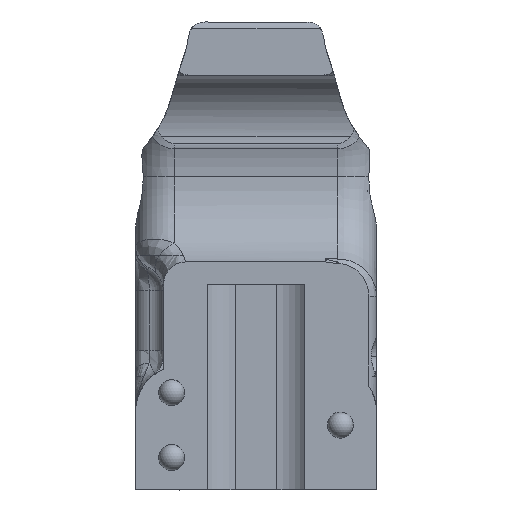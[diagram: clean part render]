
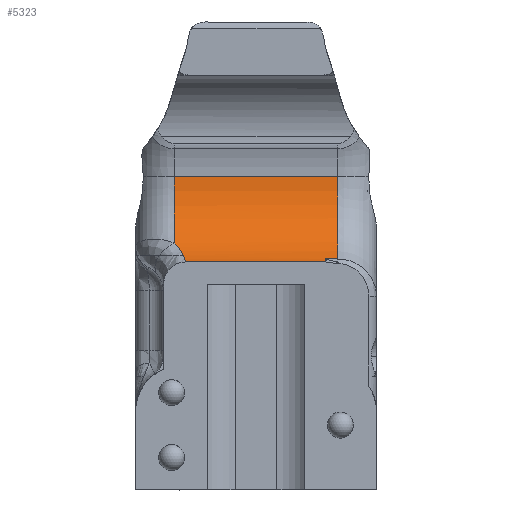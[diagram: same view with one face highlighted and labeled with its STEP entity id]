
A CAD part, left-side view. The second image highlights one B-rep face of the part: STEP entity #5323.
In plain terms, the highlighted cylindrical face has radius 14.287 mm (diameter 28.575 mm), a partial arc.
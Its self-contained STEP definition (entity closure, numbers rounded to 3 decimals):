
#4 = CARTESIAN_POINT ( 'NONE',  ( 76.653, -72.447, -1.367 ) ) ;
#103 = CARTESIAN_POINT ( 'NONE',  ( 84.171, -46.951, -13.516 ) ) ;
#279 = VERTEX_POINT ( 'NONE', #3053 ) ;
#500 = ORIENTED_EDGE ( 'NONE', *, *, #2014, .T. ) ;
#787 = CARTESIAN_POINT ( 'NONE',  ( 86.281, -45.908, -11.925 ) ) ;
#828 = LINE ( 'NONE', #6614, #8281 ) ;
#878 = EDGE_CURVE ( 'NONE', #6396, #1600, #2645, .T. ) ;
#953 = VERTEX_POINT ( 'NONE', #9269 ) ;
#1197 = CARTESIAN_POINT ( 'NONE',  ( 83.191, -72.447, -14.07 ) ) ;
#1337 = LINE ( 'NONE', #1197, #7319 ) ;
#1532 = CARTESIAN_POINT ( 'NONE',  ( 85.909, -46.184, -12.251 ) ) ;
#1600 = VERTEX_POINT ( 'NONE', #1605 ) ;
#1605 = CARTESIAN_POINT ( 'NONE',  ( 82.199, -68.875, -14.534 ) ) ;
#1796 = CIRCLE ( 'NONE', #5397, 14.288 ) ;
#1967 = EDGE_CURVE ( 'NONE', #953, #4092, #828, .T. ) ;
#2014 = EDGE_CURVE ( 'NONE', #4092, #2066, #4663, .T. ) ;
#2066 = VERTEX_POINT ( 'NONE', #3145 ) ;
#2244 = CARTESIAN_POINT ( 'NONE',  ( 85.685, -46.326, -12.437 ) ) ;
#2315 = DIRECTION ( 'NONE',  ( 0., 1., 0. ) ) ;
#2537 = CARTESIAN_POINT ( 'NONE',  ( 84.171, -46.951, -13.516 ) ) ;
#2645 = LINE ( 'NONE', #8962, #2885 ) ;
#2740 = EDGE_CURVE ( 'NONE', #1600, #279, #1796, .T. ) ;
#2885 = VECTOR ( 'NONE', #4799, 1000. ) ;
#2936 = CARTESIAN_POINT ( 'NONE',  ( 82.199, -47.274, -14.534 ) ) ;
#2976 = CARTESIAN_POINT ( 'NONE',  ( 85.556, -46.401, -12.541 ) ) ;
#3053 = CARTESIAN_POINT ( 'NONE',  ( 83.191, -68.875, -14.07 ) ) ;
#3079 = CARTESIAN_POINT ( 'NONE',  ( 76.653, -45.593, -1.367 ) ) ;
#3145 = CARTESIAN_POINT ( 'NONE',  ( 86.612, -45.593, -11.611 ) ) ;
#3301 = DIRECTION ( 'NONE',  ( 0., -1., 0. ) ) ;
#3607 = CYLINDRICAL_SURFACE ( 'NONE', #5808, 14.288 ) ;
#3700 = CARTESIAN_POINT ( 'NONE',  ( 85.515, -46.423, -12.573 ) ) ;
#3720 = DIRECTION ( 'NONE',  ( 0., -1., 0. ) ) ;
#3800 = DIRECTION ( 'NONE',  ( 1., 0., 0. ) ) ;
#4092 = VERTEX_POINT ( 'NONE', #8368 ) ;
#4126 = EDGE_CURVE ( 'NONE', #279, #5684, #1337, .T. ) ;
#4307 = ORIENTED_EDGE ( 'NONE', *, *, #8366, .T. ) ;
#4394 = CARTESIAN_POINT ( 'NONE',  ( 86.612, -45.593, -11.611 ) ) ;
#4415 = CARTESIAN_POINT ( 'NONE',  ( 84.671, -46.816, -13.206 ) ) ;
#4422 = EDGE_CURVE ( 'NONE', #2066, #7367, #6505, .T. ) ;
#4627 = CARTESIAN_POINT ( 'NONE',  ( 82.199, -47.274, -14.534 ) ) ;
#4663 = CIRCLE ( 'NONE', #9341, 14.288 ) ;
#4743 = ORIENTED_EDGE ( 'NONE', *, *, #1967, .T. ) ;
#4799 = DIRECTION ( 'NONE',  ( 0., -1., 0. ) ) ;
#4980 = ORIENTED_EDGE ( 'NONE', *, *, #4422, .T. ) ;
#5044 = DIRECTION ( 'NONE',  ( 1., 0., 0. ) ) ;
#5069 = CARTESIAN_POINT ( 'NONE',  ( 83.616, -47.101, -13.86 ) ) ;
#5323 = ADVANCED_FACE ( 'NONE', ( #9373 ), #3607, .F. ) ;
#5397 = AXIS2_PLACEMENT_3D ( 'NONE', #8046, #3720, #8779 ) ;
#5504 = DIRECTION ( 'NONE',  ( 0., -1., 0. ) ) ;
#5684 = VERTEX_POINT ( 'NONE', #7827 ) ;
#5808 = AXIS2_PLACEMENT_3D ( 'NONE', #4, #6340, #5044 ) ;
#5828 = CARTESIAN_POINT ( 'NONE',  ( 86.005, -46.117, -12.169 ) ) ;
#5846 = ORIENTED_EDGE ( 'NONE', *, *, #878, .T. ) ;
#6192 = B_SPLINE_CURVE_WITH_KNOTS ( 'NONE', 3,
 ( #7239, #5069, #7269, #2936 ),
 .UNSPECIFIED., .F., .F.,
 ( 4, 4 ),
 ( 0., 1. ),
 .UNSPECIFIED. ) ;
#6340 = DIRECTION ( 'NONE',  ( 0., 1., 0. ) ) ;
#6396 = VERTEX_POINT ( 'NONE', #4627 ) ;
#6505 = B_SPLINE_CURVE_WITH_KNOTS ( 'NONE', 3,
 ( #4394, #8721, #787, #5828, #1532, #6571, #2244, #7313, #2976, #8029, #3700, #8758, #4415, #103 ),
 .UNSPECIFIED., .F., .F.,
 ( 4, 2, 2, 1, 1, 2, 2, 4 ),
 ( 0., 0.25, 0.375, 0.437, 0.469, 0.484, 0.5, 1. ),
 .UNSPECIFIED. ) ;
#6571 = CARTESIAN_POINT ( 'NONE',  ( 85.761, -46.28, -12.375 ) ) ;
#6614 = CARTESIAN_POINT ( 'NONE',  ( 90.94, -72.447, -1.367 ) ) ;
#7145 = EDGE_LOOP ( 'NONE', ( #7271, #4743, #500, #4980, #4307, #5846, #7194, #9322 ) ) ;
#7194 = ORIENTED_EDGE ( 'NONE', *, *, #2740, .T. ) ;
#7202 = CIRCLE ( 'NONE', #8619, 14.288 ) ;
#7239 = CARTESIAN_POINT ( 'NONE',  ( 84.171, -46.951, -13.516 ) ) ;
#7269 = CARTESIAN_POINT ( 'NONE',  ( 82.962, -47.208, -14.212 ) ) ;
#7271 = ORIENTED_EDGE ( 'NONE', *, *, #7397, .T. ) ;
#7313 = CARTESIAN_POINT ( 'NONE',  ( 85.595, -46.379, -12.51 ) ) ;
#7319 = VECTOR ( 'NONE', #5504, 1000. ) ;
#7367 = VERTEX_POINT ( 'NONE', #2537 ) ;
#7397 = EDGE_CURVE ( 'NONE', #5684, #953, #7202, .T. ) ;
#7640 = CARTESIAN_POINT ( 'NONE',  ( 76.653, -70.726, -1.367 ) ) ;
#7827 = CARTESIAN_POINT ( 'NONE',  ( 83.191, -70.726, -14.07 ) ) ;
#8029 = CARTESIAN_POINT ( 'NONE',  ( 85.529, -46.415, -12.562 ) ) ;
#8046 = CARTESIAN_POINT ( 'NONE',  ( 76.653, -68.875, -1.367 ) ) ;
#8125 = DIRECTION ( 'NONE',  ( 0., 1., 0. ) ) ;
#8281 = VECTOR ( 'NONE', #2315, 1000. ) ;
#8342 = DIRECTION ( 'NONE',  ( 1., 0., 0. ) ) ;
#8366 = EDGE_CURVE ( 'NONE', #7367, #6396, #6192, .T. ) ;
#8368 = CARTESIAN_POINT ( 'NONE',  ( 90.94, -45.593, -1.367 ) ) ;
#8619 = AXIS2_PLACEMENT_3D ( 'NONE', #7640, #3301, #8342 ) ;
#8721 = CARTESIAN_POINT ( 'NONE',  ( 86.453, -45.756, -11.766 ) ) ;
#8758 = CARTESIAN_POINT ( 'NONE',  ( 85.113, -46.642, -12.89 ) ) ;
#8779 = DIRECTION ( 'NONE',  ( 1., 0., 0. ) ) ;
#8962 = CARTESIAN_POINT ( 'NONE',  ( 82.199, -72.447, -14.534 ) ) ;
#9269 = CARTESIAN_POINT ( 'NONE',  ( 90.94, -70.726, -1.367 ) ) ;
#9322 = ORIENTED_EDGE ( 'NONE', *, *, #4126, .T. ) ;
#9341 = AXIS2_PLACEMENT_3D ( 'NONE', #3079, #8125, #3800 ) ;
#9373 = FACE_OUTER_BOUND ( 'NONE', #7145, .T. ) ;
